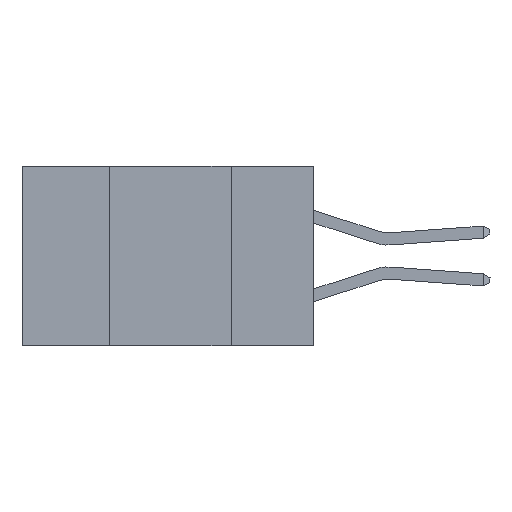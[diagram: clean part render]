
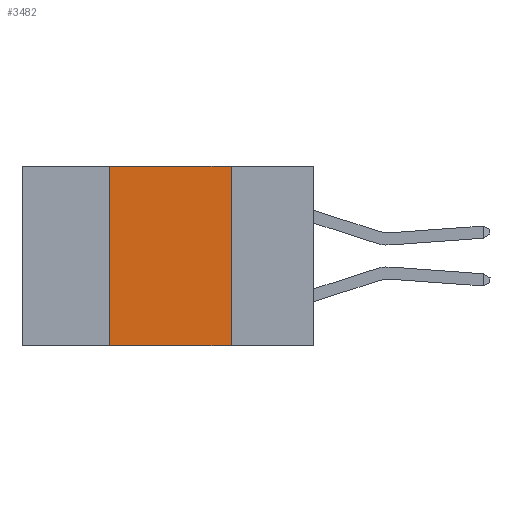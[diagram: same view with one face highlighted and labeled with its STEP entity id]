
A CAD part, left-side view. The second image highlights one B-rep face of the part: STEP entity #3482.
In plain terms, the highlighted planar face has unit normal (-1, 0, 0).
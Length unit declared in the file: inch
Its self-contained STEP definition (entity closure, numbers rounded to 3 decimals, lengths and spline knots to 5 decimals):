
#472 = EDGE_CURVE ( 'NONE', #21147, #1936, #4405, .T. ) ;
#675 = ORIENTED_EDGE ( 'NONE', *, *, #472, .F. ) ;
#1805 = VECTOR ( 'NONE', #10349, 39.37008 ) ;
#1936 = VERTEX_POINT ( 'NONE', #11395 ) ;
#3426 = LINE ( 'NONE', #19216, #14665 ) ;
#3482 = ADVANCED_FACE ( 'NONE', ( #20571 ), #5334, .F. ) ;
#4019 = EDGE_CURVE ( 'NONE', #7027, #11531, #3426, .T. ) ;
#4169 = VECTOR ( 'NONE', #7433, 39.37008 ) ;
#4405 = LINE ( 'NONE', #4633, #6558 ) ;
#4633 = CARTESIAN_POINT ( 'NONE',  ( 0., 0.42, 0. ) ) ;
#5334 = PLANE ( 'NONE',  #22037 ) ;
#5707 = CARTESIAN_POINT ( 'NONE',  ( 0., 0.6, 0. ) ) ;
#6043 = LINE ( 'NONE', #5707, #4169 ) ;
#6066 = LINE ( 'NONE', #8560, #1805 ) ;
#6135 = EDGE_CURVE ( 'NONE', #1936, #7027, #6043, .T. ) ;
#6558 = VECTOR ( 'NONE', #6972, 39.37008 ) ;
#6972 = DIRECTION ( 'NONE',  ( 0., 0., 1. ) ) ;
#7027 = VERTEX_POINT ( 'NONE', #18000 ) ;
#7433 = DIRECTION ( 'NONE',  ( 0., -1., 0. ) ) ;
#7741 = ORIENTED_EDGE ( 'NONE', *, *, #6135, .F. ) ;
#8255 = ORIENTED_EDGE ( 'NONE', *, *, #4019, .F. ) ;
#8560 = CARTESIAN_POINT ( 'NONE',  ( 0., 0.6, -0.37 ) ) ;
#8992 = DIRECTION ( 'NONE',  ( 0., 0., -1. ) ) ;
#9014 = DIRECTION ( 'NONE',  ( 1., 0., 0. ) ) ;
#10349 = DIRECTION ( 'NONE',  ( 0., -1., 0. ) ) ;
#11254 = ORIENTED_EDGE ( 'NONE', *, *, #11379, .T. ) ;
#11379 = EDGE_CURVE ( 'NONE', #21147, #11531, #6066, .T. ) ;
#11395 = CARTESIAN_POINT ( 'NONE',  ( 0., 0.42, 0. ) ) ;
#11531 = VERTEX_POINT ( 'NONE', #21710 ) ;
#12265 = DIRECTION ( 'NONE',  ( 0., 0., -1. ) ) ;
#12333 = CARTESIAN_POINT ( 'NONE',  ( 0., 0.6, 0. ) ) ;
#13727 = CARTESIAN_POINT ( 'NONE',  ( 0., 0.42, -0.37 ) ) ;
#14665 = VECTOR ( 'NONE', #8992, 39.37008 ) ;
#16495 = EDGE_LOOP ( 'NONE', ( #8255, #7741, #675, #11254 ) ) ;
#18000 = CARTESIAN_POINT ( 'NONE',  ( 0., 0.17, 0. ) ) ;
#19216 = CARTESIAN_POINT ( 'NONE',  ( 0., 0.17, 0. ) ) ;
#20571 = FACE_OUTER_BOUND ( 'NONE', #16495, .T. ) ;
#21147 = VERTEX_POINT ( 'NONE', #13727 ) ;
#21710 = CARTESIAN_POINT ( 'NONE',  ( 0., 0.17, -0.37 ) ) ;
#22037 = AXIS2_PLACEMENT_3D ( 'NONE', #12333, #9014, #12265 ) ;
